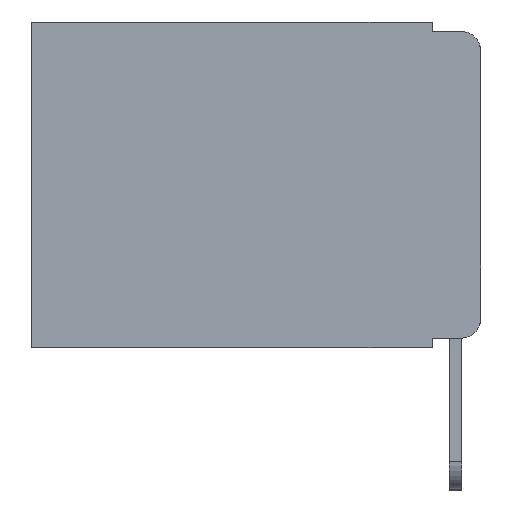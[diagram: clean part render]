
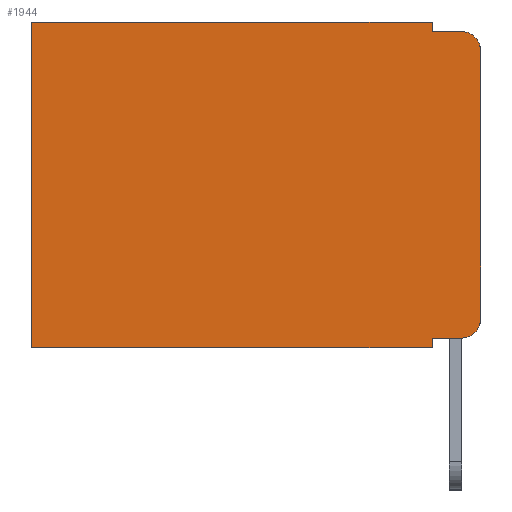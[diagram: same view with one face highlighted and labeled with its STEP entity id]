
A CAD part, left-side view. The second image highlights one B-rep face of the part: STEP entity #1944.
In plain terms, the highlighted planar face has unit normal (-1, 0, 0).
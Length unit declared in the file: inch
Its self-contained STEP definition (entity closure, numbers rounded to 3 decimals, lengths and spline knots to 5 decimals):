
#1 = EDGE_CURVE ( 'NONE', #10608, #1692, #1551, .T. ) ;
#26 = EDGE_CURVE ( 'NONE', #4844, #1053, #4179, .T. ) ;
#536 = DIRECTION ( 'NONE',  ( -1., 0., 0. ) ) ;
#1037 = AXIS2_PLACEMENT_3D ( 'NONE', #8125, #8088, #10418 ) ;
#1053 = VERTEX_POINT ( 'NONE', #1522 ) ;
#1217 = VERTEX_POINT ( 'NONE', #6064 ) ;
#1223 = PLANE ( 'NONE',  #3466 ) ;
#1277 = CARTESIAN_POINT ( 'NONE',  ( 0.298, 0.473, 0. ) ) ;
#1349 = EDGE_CURVE ( 'NONE', #6687, #1217, #5535, .T. ) ;
#1522 = CARTESIAN_POINT ( 'NONE',  ( 0.298, 0.051, -0.01 ) ) ;
#1551 = LINE ( 'NONE', #9417, #12071 ) ;
#1637 = CARTESIAN_POINT ( 'NONE',  ( 0.298, 0.051, -0.333 ) ) ;
#1692 = VERTEX_POINT ( 'NONE', #10340 ) ;
#1930 = VECTOR ( 'NONE', #12305, 39.37008 ) ;
#1944 = ADVANCED_FACE ( 'NONE', ( #3263 ), #1223, .F. ) ;
#2313 = VECTOR ( 'NONE', #8576, 39.37008 ) ;
#2489 = CIRCLE ( 'NONE', #1037, 0.02 ) ;
#2617 = EDGE_CURVE ( 'NONE', #6687, #4039, #2489, .T. ) ;
#2779 = EDGE_CURVE ( 'NONE', #9984, #3086, #8129, .T. ) ;
#2920 = DIRECTION ( 'NONE',  ( 0., -1., 0. ) ) ;
#3064 = CARTESIAN_POINT ( 'NONE',  ( 0.298, 0., 0. ) ) ;
#3079 = CARTESIAN_POINT ( 'NONE',  ( 0.298, 0., 0. ) ) ;
#3086 = VERTEX_POINT ( 'NONE', #12785 ) ;
#3182 = EDGE_CURVE ( 'NONE', #4844, #9916, #9783, .T. ) ;
#3263 = FACE_OUTER_BOUND ( 'NONE', #5715, .T. ) ;
#3466 = AXIS2_PLACEMENT_3D ( 'NONE', #3064, #11515, #6451 ) ;
#4039 = VERTEX_POINT ( 'NONE', #8710 ) ;
#4179 = LINE ( 'NONE', #9183, #11465 ) ;
#4844 = VERTEX_POINT ( 'NONE', #7870 ) ;
#4849 = ORIENTED_EDGE ( 'NONE', *, *, #6434, .T. ) ;
#4945 = CARTESIAN_POINT ( 'NONE',  ( 0.298, 0.051, -0.343 ) ) ;
#5101 = DIRECTION ( 'NONE',  ( 0., 0., -1. ) ) ;
#5333 = CARTESIAN_POINT ( 'NONE',  ( 0.298, 0., 0. ) ) ;
#5535 = LINE ( 'NONE', #5333, #10504 ) ;
#5670 = LINE ( 'NONE', #6530, #13133 ) ;
#5715 = EDGE_LOOP ( 'NONE', ( #7316, #7550, #7534, #7614, #7682, #7671, #7726, #7747, #7863, #4849 ) ) ;
#5787 = DIRECTION ( 'NONE',  ( 0., 1., 0. ) ) ;
#6064 = CARTESIAN_POINT ( 'NONE',  ( 0.298, 0., -0.313 ) ) ;
#6088 = LINE ( 'NONE', #1277, #8740 ) ;
#6160 = CARTESIAN_POINT ( 'NONE',  ( 0.298, 0., -0.03 ) ) ;
#6434 = EDGE_CURVE ( 'NONE', #3086, #1217, #12754, .T. ) ;
#6451 = DIRECTION ( 'NONE',  ( 0., 0., -1. ) ) ;
#6530 = CARTESIAN_POINT ( 'NONE',  ( 0.298, 0.051, 0. ) ) ;
#6687 = VERTEX_POINT ( 'NONE', #6160 ) ;
#6924 = CARTESIAN_POINT ( 'NONE',  ( 0.298, 0.02, -0.313 ) ) ;
#6935 = EDGE_CURVE ( 'NONE', #9984, #10608, #5670, .T. ) ;
#7316 = ORIENTED_EDGE ( 'NONE', *, *, #1349, .F. ) ;
#7534 = ORIENTED_EDGE ( 'NONE', *, *, #8025, .F. ) ;
#7550 = ORIENTED_EDGE ( 'NONE', *, *, #2617, .T. ) ;
#7614 = ORIENTED_EDGE ( 'NONE', *, *, #26, .F. ) ;
#7671 = ORIENTED_EDGE ( 'NONE', *, *, #8463, .T. ) ;
#7682 = ORIENTED_EDGE ( 'NONE', *, *, #3182, .T. ) ;
#7726 = ORIENTED_EDGE ( 'NONE', *, *, #1, .F. ) ;
#7747 = ORIENTED_EDGE ( 'NONE', *, *, #6935, .F. ) ;
#7863 = ORIENTED_EDGE ( 'NONE', *, *, #2779, .T. ) ;
#7870 = CARTESIAN_POINT ( 'NONE',  ( 0.298, 0.051, 0. ) ) ;
#8025 = EDGE_CURVE ( 'NONE', #1053, #4039, #10440, .T. ) ;
#8088 = DIRECTION ( 'NONE',  ( -1., 0., 0. ) ) ;
#8125 = CARTESIAN_POINT ( 'NONE',  ( 0.298, 0.02, -0.03 ) ) ;
#8129 = LINE ( 'NONE', #8610, #2313 ) ;
#8463 = EDGE_CURVE ( 'NONE', #9916, #1692, #6088, .T. ) ;
#8576 = DIRECTION ( 'NONE',  ( 0., -1., 0. ) ) ;
#8610 = CARTESIAN_POINT ( 'NONE',  ( 0.298, 0.051, -0.333 ) ) ;
#8710 = CARTESIAN_POINT ( 'NONE',  ( 0.298, 0.02, -0.01 ) ) ;
#8740 = VECTOR ( 'NONE', #12448, 39.37008 ) ;
#8963 = DIRECTION ( 'NONE',  ( 0., 0., -1. ) ) ;
#8991 = CARTESIAN_POINT ( 'NONE',  ( 0.298, 0.051, -0.01 ) ) ;
#9183 = CARTESIAN_POINT ( 'NONE',  ( 0.298, 0.051, 0. ) ) ;
#9417 = CARTESIAN_POINT ( 'NONE',  ( 0.298, 0., -0.343 ) ) ;
#9485 = DIRECTION ( 'NONE',  ( 0., 0., -1. ) ) ;
#9783 = LINE ( 'NONE', #3079, #1930 ) ;
#9916 = VERTEX_POINT ( 'NONE', #11755 ) ;
#9984 = VERTEX_POINT ( 'NONE', #1637 ) ;
#10340 = CARTESIAN_POINT ( 'NONE',  ( 0.298, 0.473, -0.343 ) ) ;
#10418 = DIRECTION ( 'NONE',  ( 0., 0., -1. ) ) ;
#10440 = LINE ( 'NONE', #8991, #12988 ) ;
#10504 = VECTOR ( 'NONE', #5101, 39.37008 ) ;
#10608 = VERTEX_POINT ( 'NONE', #4945 ) ;
#11465 = VECTOR ( 'NONE', #12090, 39.37008 ) ;
#11468 = AXIS2_PLACEMENT_3D ( 'NONE', #6924, #536, #8963 ) ;
#11515 = DIRECTION ( 'NONE',  ( 1., 0., 0. ) ) ;
#11755 = CARTESIAN_POINT ( 'NONE',  ( 0.298, 0.473, 0. ) ) ;
#12071 = VECTOR ( 'NONE', #5787, 39.37008 ) ;
#12090 = DIRECTION ( 'NONE',  ( 0., 0., -1. ) ) ;
#12305 = DIRECTION ( 'NONE',  ( 0., 1., 0. ) ) ;
#12448 = DIRECTION ( 'NONE',  ( 0., 0., -1. ) ) ;
#12754 = CIRCLE ( 'NONE', #11468, 0.02 ) ;
#12785 = CARTESIAN_POINT ( 'NONE',  ( 0.298, 0.02, -0.333 ) ) ;
#12988 = VECTOR ( 'NONE', #2920, 39.37008 ) ;
#13133 = VECTOR ( 'NONE', #9485, 39.37008 ) ;
